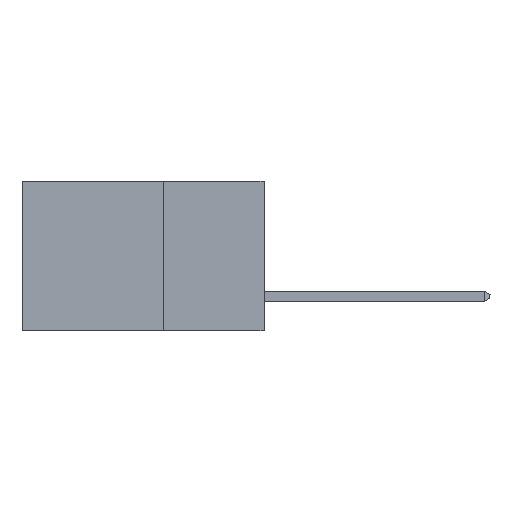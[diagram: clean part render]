
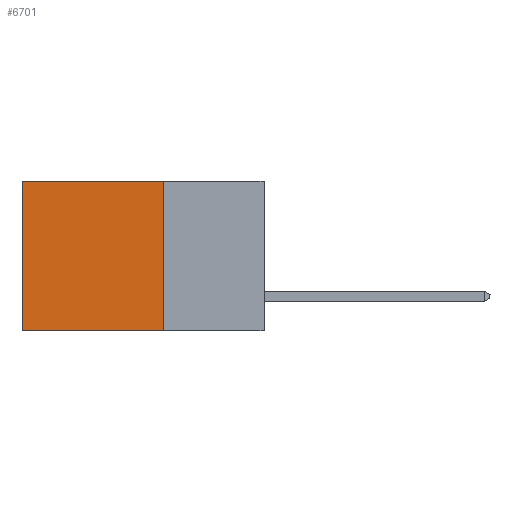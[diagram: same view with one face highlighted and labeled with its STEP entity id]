
A CAD part, left-side view. The second image highlights one B-rep face of the part: STEP entity #6701.
In plain terms, the highlighted planar face has unit normal (-1, 0, 0).
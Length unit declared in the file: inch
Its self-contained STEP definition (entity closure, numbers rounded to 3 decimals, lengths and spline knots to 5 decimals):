
#191 = EDGE_LOOP ( 'NONE', ( #15302, #6210, #19206, #22505 ) ) ;
#570 = DIRECTION ( 'NONE',  ( 0., 0., -1. ) ) ;
#957 = CARTESIAN_POINT ( 'NONE',  ( 0.2615, 0.25, -0.37 ) ) ;
#2361 = PLANE ( 'NONE',  #4634 ) ;
#3101 = DIRECTION ( 'NONE',  ( 0., 0., -1. ) ) ;
#3358 = EDGE_CURVE ( 'NONE', #8703, #12995, #18866, .T. ) ;
#4000 = FACE_OUTER_BOUND ( 'NONE', #191, .T. ) ;
#4634 = AXIS2_PLACEMENT_3D ( 'NONE', #9144, #21820, #570 ) ;
#5070 = CARTESIAN_POINT ( 'NONE',  ( 0.2615, 0.6, -0.37 ) ) ;
#5829 = VECTOR ( 'NONE', #16537, 39.37008 ) ;
#6210 = ORIENTED_EDGE ( 'NONE', *, *, #3358, .F. ) ;
#6701 = ADVANCED_FACE ( 'NONE', ( #4000 ), #2361, .F. ) ;
#6805 = LINE ( 'NONE', #5070, #22687 ) ;
#7182 = CARTESIAN_POINT ( 'NONE',  ( 0.2615, 0.25, 0. ) ) ;
#7281 = CARTESIAN_POINT ( 'NONE',  ( 0.2615, 0.6, -0.37 ) ) ;
#7688 = CARTESIAN_POINT ( 'NONE',  ( 0.2615, 0.25, 0. ) ) ;
#7876 = EDGE_CURVE ( 'NONE', #16039, #8703, #10611, .T. ) ;
#8237 = DIRECTION ( 'NONE',  ( 0., 1., 0. ) ) ;
#8260 = VECTOR ( 'NONE', #8237, 39.37008 ) ;
#8703 = VERTEX_POINT ( 'NONE', #10517 ) ;
#9144 = CARTESIAN_POINT ( 'NONE',  ( 0.2615, 0.25, -0.37 ) ) ;
#10517 = CARTESIAN_POINT ( 'NONE',  ( 0.2615, 0.25, -0.37 ) ) ;
#10611 = LINE ( 'NONE', #19946, #5829 ) ;
#10887 = DIRECTION ( 'NONE',  ( 0., 1., 0. ) ) ;
#12204 = EDGE_CURVE ( 'NONE', #16039, #17528, #21911, .T. ) ;
#12995 = VERTEX_POINT ( 'NONE', #7281 ) ;
#15302 = ORIENTED_EDGE ( 'NONE', *, *, #18045, .T. ) ;
#16039 = VERTEX_POINT ( 'NONE', #7182 ) ;
#16114 = VECTOR ( 'NONE', #10887, 39.37008 ) ;
#16537 = DIRECTION ( 'NONE',  ( 0., 0., -1. ) ) ;
#17528 = VERTEX_POINT ( 'NONE', #22441 ) ;
#18045 = EDGE_CURVE ( 'NONE', #17528, #12995, #6805, .T. ) ;
#18866 = LINE ( 'NONE', #957, #8260 ) ;
#19206 = ORIENTED_EDGE ( 'NONE', *, *, #7876, .F. ) ;
#19946 = CARTESIAN_POINT ( 'NONE',  ( 0.2615, 0.25, -0.37 ) ) ;
#21820 = DIRECTION ( 'NONE',  ( 1., 0., 0. ) ) ;
#21911 = LINE ( 'NONE', #7688, #16114 ) ;
#22441 = CARTESIAN_POINT ( 'NONE',  ( 0.2615, 0.6, 0. ) ) ;
#22505 = ORIENTED_EDGE ( 'NONE', *, *, #12204, .T. ) ;
#22687 = VECTOR ( 'NONE', #3101, 39.37008 ) ;
